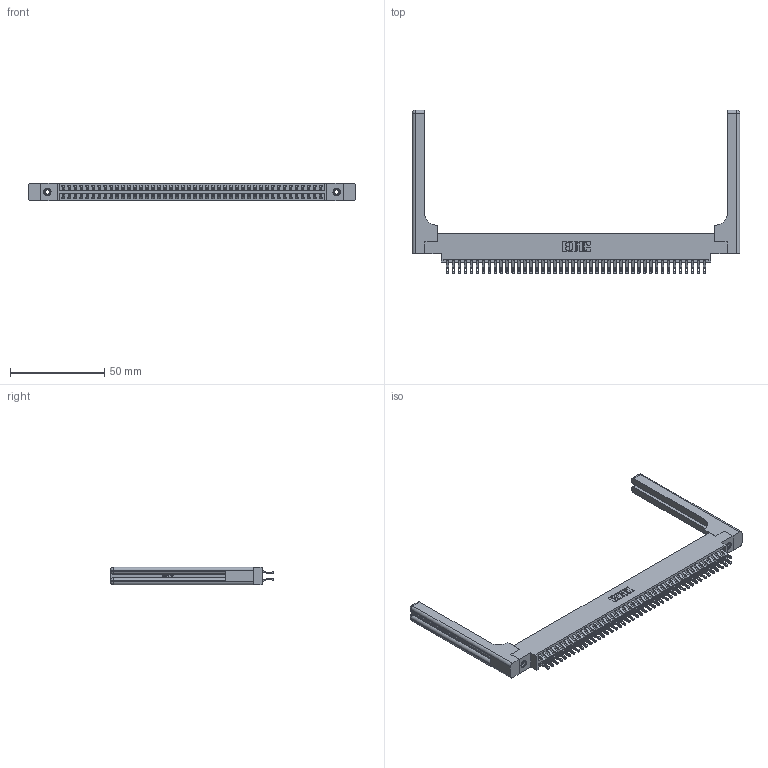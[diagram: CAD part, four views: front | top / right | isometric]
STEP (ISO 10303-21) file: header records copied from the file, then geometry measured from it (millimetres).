
FILE_DESCRIPTION (( 'STEP AP203' ), '1' );
FILE_NAME ('396-088-555-858.STEP', '2019-11-02T15:15:33', ( '' ), ( '' ), 'SwSTEP 2.0', 'SolidWorks 2016', '' );
FILE_SCHEMA (( 'CONFIG_CONTROL_DESIGN' ));
Length unit declared in the file: inch
Products named in the file (5): 346 Part_0.170 Offset - 0.156 Dia-TH; 345-292-001_555 Tail; 345-250-001_345-250-001-102; 346-220-058_345-220-058; 396-088-555-858
Assembly tree (93 placements, depth 2):
  396-088-555-858
    346 Part_0.170 Offset - 0.156 Dia-TH
    345-292-001_555 Tail  x88
    345-250-001_345-250-001-102  x2
    346-220-058_345-220-058  x2
Bounding box: 173.76 x 86.74 x 9.4 mm (x, y, z)
Volume: 24554.3 mm3; surface area: 29543.9 mm2
Topology: 93 solids, 93 shells, 5486 faces, 17111 edges, 11386 vertices
Faces by surface type: plane 3132, cylinder 2294, bspline 36, cone 12, sphere 8, torus 4
Entity records: 34086 total; most frequent: CARTESIAN_POINT 6659, ORIENTED_EDGE 5360, DIRECTION 4820, EDGE_CURVE 2680, LINE 2260, VECTOR 2260, VERTEX_POINT 1778, AXIS2_PLACEMENT_3D 1280
